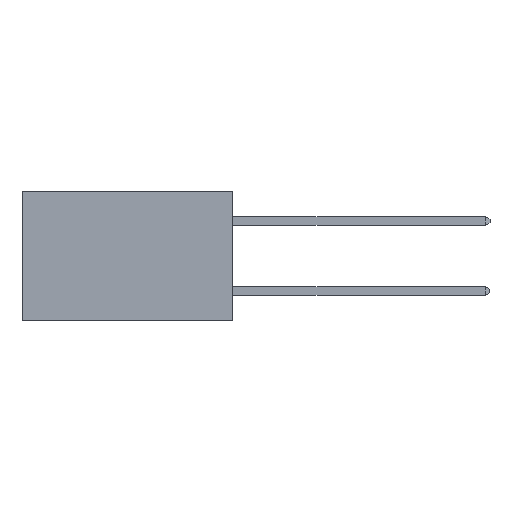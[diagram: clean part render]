
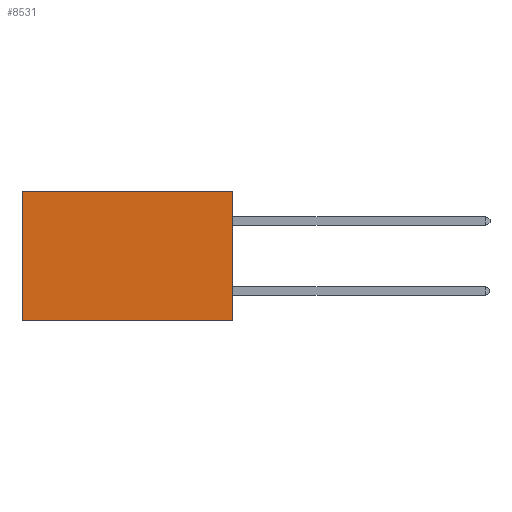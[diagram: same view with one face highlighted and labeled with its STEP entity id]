
A CAD part, left-side view. The second image highlights one B-rep face of the part: STEP entity #8531.
In plain terms, the highlighted planar face has unit normal (-1, 0, 0).
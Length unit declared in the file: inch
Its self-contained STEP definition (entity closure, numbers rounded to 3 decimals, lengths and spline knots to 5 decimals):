
#812 = ORIENTED_EDGE ( 'NONE', *, *, #10701, .T. ) ;
#836 = DIRECTION ( 'NONE',  ( 0., 1., 0. ) ) ;
#1155 = VECTOR ( 'NONE', #836, 39.37008 ) ;
#1688 = LINE ( 'NONE', #1796, #2006 ) ;
#1773 = VERTEX_POINT ( 'NONE', #7249 ) ;
#1796 = CARTESIAN_POINT ( 'NONE',  ( 0.2875, 0.6, 0. ) ) ;
#2006 = VECTOR ( 'NONE', #2294, 39.37008 ) ;
#2115 = AXIS2_PLACEMENT_3D ( 'NONE', #5307, #3537, #9528 ) ;
#2263 = EDGE_CURVE ( 'NONE', #4773, #5321, #1688, .T. ) ;
#2294 = DIRECTION ( 'NONE',  ( 0., 0., -1. ) ) ;
#2609 = CARTESIAN_POINT ( 'NONE',  ( 0.2875, 0., 0. ) ) ;
#3537 = DIRECTION ( 'NONE',  ( 1., 0., 0. ) ) ;
#3915 = LINE ( 'NONE', #11185, #1155 ) ;
#3988 = VERTEX_POINT ( 'NONE', #4147 ) ;
#4147 = CARTESIAN_POINT ( 'NONE',  ( 0.2875, 0., 0. ) ) ;
#4193 = ORIENTED_EDGE ( 'NONE', *, *, #7739, .F. ) ;
#4406 = DIRECTION ( 'NONE',  ( 0., 1., 0. ) ) ;
#4773 = VERTEX_POINT ( 'NONE', #8943 ) ;
#5307 = CARTESIAN_POINT ( 'NONE',  ( 0.2875, 0., 0. ) ) ;
#5321 = VERTEX_POINT ( 'NONE', #9576 ) ;
#5575 = DIRECTION ( 'NONE',  ( 0., 0., -1. ) ) ;
#6404 = ORIENTED_EDGE ( 'NONE', *, *, #8574, .F. ) ;
#6734 = LINE ( 'NONE', #2609, #10877 ) ;
#7249 = CARTESIAN_POINT ( 'NONE',  ( 0.2875, 0., -0.37 ) ) ;
#7265 = EDGE_LOOP ( 'NONE', ( #9282, #6404, #4193, #812 ) ) ;
#7739 = EDGE_CURVE ( 'NONE', #3988, #1773, #10008, .T. ) ;
#7827 = VECTOR ( 'NONE', #5575, 39.37008 ) ;
#8531 = ADVANCED_FACE ( 'NONE', ( #8727 ), #8695, .F. ) ;
#8574 = EDGE_CURVE ( 'NONE', #1773, #5321, #3915, .T. ) ;
#8695 = PLANE ( 'NONE',  #2115 ) ;
#8727 = FACE_OUTER_BOUND ( 'NONE', #7265, .T. ) ;
#8783 = CARTESIAN_POINT ( 'NONE',  ( 0.2875, 0., 0. ) ) ;
#8943 = CARTESIAN_POINT ( 'NONE',  ( 0.2875, 0.6, 0. ) ) ;
#9282 = ORIENTED_EDGE ( 'NONE', *, *, #2263, .T. ) ;
#9528 = DIRECTION ( 'NONE',  ( 0., 0., -1. ) ) ;
#9576 = CARTESIAN_POINT ( 'NONE',  ( 0.2875, 0.6, -0.37 ) ) ;
#10008 = LINE ( 'NONE', #8783, #7827 ) ;
#10701 = EDGE_CURVE ( 'NONE', #3988, #4773, #6734, .T. ) ;
#10877 = VECTOR ( 'NONE', #4406, 39.37008 ) ;
#11185 = CARTESIAN_POINT ( 'NONE',  ( 0.2875, 0., -0.37 ) ) ;
